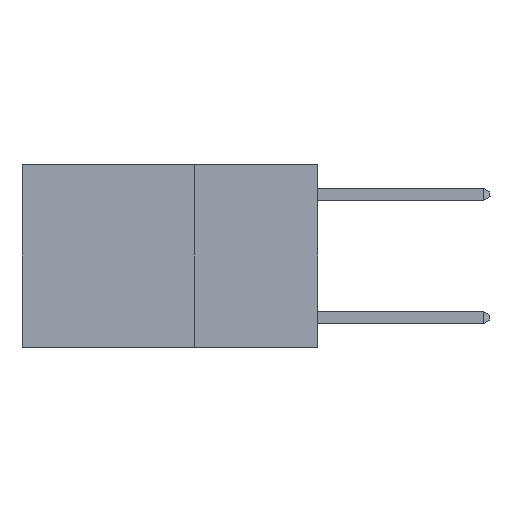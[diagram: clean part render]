
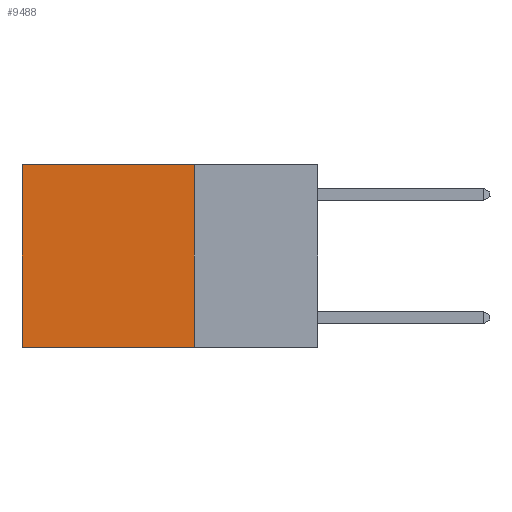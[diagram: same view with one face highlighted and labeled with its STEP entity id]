
A CAD part, left-side view. The second image highlights one B-rep face of the part: STEP entity #9488.
In plain terms, the highlighted planar face has unit normal (-1, 0, 0).
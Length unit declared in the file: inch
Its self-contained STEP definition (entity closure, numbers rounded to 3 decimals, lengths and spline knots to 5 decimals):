
#380 = LINE ( 'NONE', #1912, #6542 ) ;
#399 = CARTESIAN_POINT ( 'NONE',  ( 0.2625, 0.6, -0.37 ) ) ;
#804 = DIRECTION ( 'NONE',  ( 0., 1., 0. ) ) ;
#905 = DIRECTION ( 'NONE',  ( 0., 0., -1. ) ) ;
#1218 = VERTEX_POINT ( 'NONE', #12496 ) ;
#1912 = CARTESIAN_POINT ( 'NONE',  ( 0.2625, 0.25, 0. ) ) ;
#2026 = CARTESIAN_POINT ( 'NONE',  ( 0.2625, 0.25, 0. ) ) ;
#2174 = VECTOR ( 'NONE', #905, 39.37008 ) ;
#2295 = ORIENTED_EDGE ( 'NONE', *, *, #13057, .T. ) ;
#2487 = VERTEX_POINT ( 'NONE', #399 ) ;
#2632 = DIRECTION ( 'NONE',  ( 0., 1., 0. ) ) ;
#3099 = DIRECTION ( 'NONE',  ( 0., 0., -1. ) ) ;
#3128 = VECTOR ( 'NONE', #2632, 39.37008 ) ;
#3211 = DIRECTION ( 'NONE',  ( 1., 0., 0. ) ) ;
#3413 = EDGE_LOOP ( 'NONE', ( #2295, #14148, #4988, #9958 ) ) ;
#4490 = CARTESIAN_POINT ( 'NONE',  ( 0.2625, 0.6, 0. ) ) ;
#4642 = VECTOR ( 'NONE', #804, 39.37008 ) ;
#4737 = AXIS2_PLACEMENT_3D ( 'NONE', #2026, #3211, #11188 ) ;
#4774 = VERTEX_POINT ( 'NONE', #11392 ) ;
#4988 = ORIENTED_EDGE ( 'NONE', *, *, #6577, .F. ) ;
#5230 = LINE ( 'NONE', #4490, #2174 ) ;
#6117 = LINE ( 'NONE', #9413, #3128 ) ;
#6542 = VECTOR ( 'NONE', #3099, 39.37008 ) ;
#6577 = EDGE_CURVE ( 'NONE', #1218, #4774, #380, .T. ) ;
#6602 = VERTEX_POINT ( 'NONE', #7580 ) ;
#7137 = FACE_OUTER_BOUND ( 'NONE', #3413, .T. ) ;
#7530 = EDGE_CURVE ( 'NONE', #4774, #2487, #13746, .T. ) ;
#7580 = CARTESIAN_POINT ( 'NONE',  ( 0.2625, 0.6, 0. ) ) ;
#8787 = PLANE ( 'NONE',  #4737 ) ;
#9413 = CARTESIAN_POINT ( 'NONE',  ( 0.2625, 0.25, 0. ) ) ;
#9488 = ADVANCED_FACE ( 'NONE', ( #7137 ), #8787, .F. ) ;
#9958 = ORIENTED_EDGE ( 'NONE', *, *, #11630, .T. ) ;
#11188 = DIRECTION ( 'NONE',  ( 0., 0., -1. ) ) ;
#11392 = CARTESIAN_POINT ( 'NONE',  ( 0.2625, 0.25, -0.37 ) ) ;
#11630 = EDGE_CURVE ( 'NONE', #1218, #6602, #6117, .T. ) ;
#12496 = CARTESIAN_POINT ( 'NONE',  ( 0.2625, 0.25, 0. ) ) ;
#13057 = EDGE_CURVE ( 'NONE', #6602, #2487, #5230, .T. ) ;
#13444 = CARTESIAN_POINT ( 'NONE',  ( 0.2625, 0.25, -0.37 ) ) ;
#13746 = LINE ( 'NONE', #13444, #4642 ) ;
#14148 = ORIENTED_EDGE ( 'NONE', *, *, #7530, .F. ) ;
